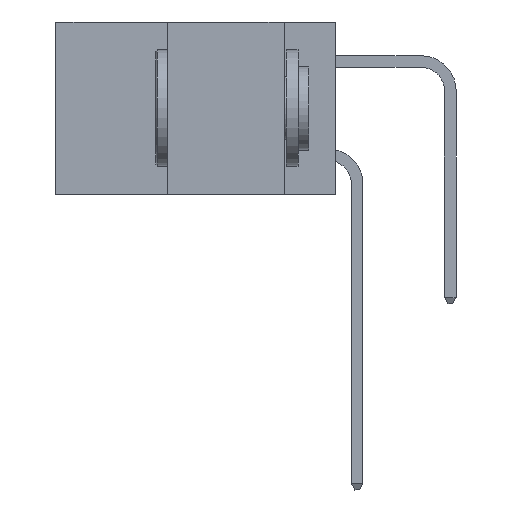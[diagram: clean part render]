
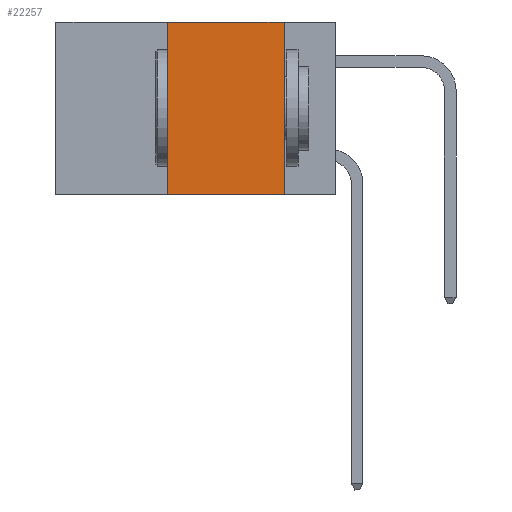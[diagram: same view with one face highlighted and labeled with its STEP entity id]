
A CAD part, left-side view. The second image highlights one B-rep face of the part: STEP entity #22257.
In plain terms, the highlighted planar face has unit normal (-1, 0, 0).
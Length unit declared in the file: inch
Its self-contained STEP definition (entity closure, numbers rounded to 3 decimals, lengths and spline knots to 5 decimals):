
#1303 = VERTEX_POINT ( 'NONE', #6830 ) ;
#1912 = ORIENTED_EDGE ( 'NONE', *, *, #23121, .F. ) ;
#2757 = DIRECTION ( 'NONE',  ( 1., 0., 0. ) ) ;
#3773 = CARTESIAN_POINT ( 'NONE',  ( 0., 0.11, 0. ) ) ;
#3975 = VECTOR ( 'NONE', #35630, 39.37008 ) ;
#4544 = CARTESIAN_POINT ( 'NONE',  ( 0., 0.36, -0.37 ) ) ;
#5432 = ORIENTED_EDGE ( 'NONE', *, *, #30174, .T. ) ;
#5883 = AXIS2_PLACEMENT_3D ( 'NONE', #39068, #2757, #24248 ) ;
#6405 = DIRECTION ( 'NONE',  ( 0., -1., 0. ) ) ;
#6830 = CARTESIAN_POINT ( 'NONE',  ( 0., 0.11, -0.37 ) ) ;
#7352 = FACE_OUTER_BOUND ( 'NONE', #38178, .T. ) ;
#7439 = CARTESIAN_POINT ( 'NONE',  ( 0., 0.36, 0. ) ) ;
#9895 = VERTEX_POINT ( 'NONE', #12531 ) ;
#10006 = VERTEX_POINT ( 'NONE', #3773 ) ;
#10164 = VERTEX_POINT ( 'NONE', #4544 ) ;
#11210 = CARTESIAN_POINT ( 'NONE',  ( 0., 0.11, 0. ) ) ;
#12531 = CARTESIAN_POINT ( 'NONE',  ( 0., 0.36, 0. ) ) ;
#13293 = VECTOR ( 'NONE', #23542, 39.37008 ) ;
#15561 = CARTESIAN_POINT ( 'NONE',  ( 0., 0.6, 0. ) ) ;
#16850 = ORIENTED_EDGE ( 'NONE', *, *, #18183, .F. ) ;
#16969 = LINE ( 'NONE', #7439, #24120 ) ;
#18183 = EDGE_CURVE ( 'NONE', #9895, #10006, #35915, .T. ) ;
#19672 = DIRECTION ( 'NONE',  ( 0., 0., 1. ) ) ;
#20554 = CARTESIAN_POINT ( 'NONE',  ( 0., 0.6, -0.37 ) ) ;
#21198 = PLANE ( 'NONE',  #5883 ) ;
#21448 = LINE ( 'NONE', #11210, #13293 ) ;
#22257 = ADVANCED_FACE ( 'NONE', ( #7352 ), #21198, .F. ) ;
#23121 = EDGE_CURVE ( 'NONE', #10164, #9895, #16969, .T. ) ;
#23542 = DIRECTION ( 'NONE',  ( 0., 0., -1. ) ) ;
#24120 = VECTOR ( 'NONE', #19672, 39.37008 ) ;
#24248 = DIRECTION ( 'NONE',  ( 0., 0., -1. ) ) ;
#27712 = EDGE_CURVE ( 'NONE', #10006, #1303, #21448, .T. ) ;
#28419 = LINE ( 'NONE', #20554, #3975 ) ;
#30174 = EDGE_CURVE ( 'NONE', #10164, #1303, #28419, .T. ) ;
#32423 = ORIENTED_EDGE ( 'NONE', *, *, #27712, .F. ) ;
#34975 = VECTOR ( 'NONE', #6405, 39.37008 ) ;
#35630 = DIRECTION ( 'NONE',  ( 0., -1., 0. ) ) ;
#35915 = LINE ( 'NONE', #15561, #34975 ) ;
#38178 = EDGE_LOOP ( 'NONE', ( #32423, #16850, #1912, #5432 ) ) ;
#39068 = CARTESIAN_POINT ( 'NONE',  ( 0., 0.6, 0. ) ) ;
